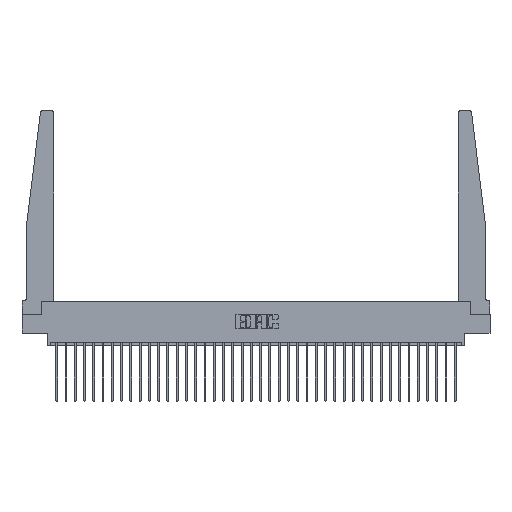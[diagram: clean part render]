
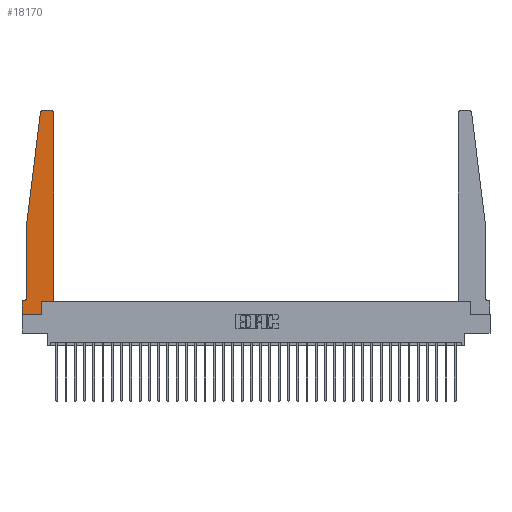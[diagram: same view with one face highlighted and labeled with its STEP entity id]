
A CAD part, top view. The second image highlights one B-rep face of the part: STEP entity #18170.
In plain terms, the highlighted planar face has unit normal (0, 0, 1).
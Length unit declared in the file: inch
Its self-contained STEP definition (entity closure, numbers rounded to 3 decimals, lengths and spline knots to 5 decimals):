
#316 = EDGE_CURVE ( 'NONE', #16473, #30556, #5155, .T. ) ;
#1388 = AXIS2_PLACEMENT_3D ( 'NONE', #4182, #32562, #17225 ) ;
#1612 = VECTOR ( 'NONE', #4434, 39.37008 ) ;
#2381 = ORIENTED_EDGE ( 'NONE', *, *, #28974, .T. ) ;
#2939 = CIRCLE ( 'NONE', #5296, 0.03 ) ;
#3600 = VERTEX_POINT ( 'NONE', #17891 ) ;
#3650 = CARTESIAN_POINT ( 'NONE',  ( 0., 0., 0.37 ) ) ;
#4142 = CARTESIAN_POINT ( 'NONE',  ( 0.425, 0.18, 0.37 ) ) ;
#4182 = CARTESIAN_POINT ( 'NONE',  ( 0., 0.1875, 0.37 ) ) ;
#4259 = VERTEX_POINT ( 'NONE', #17945 ) ;
#4434 = DIRECTION ( 'NONE',  ( -0.122, -0.992, 0. ) ) ;
#4478 = VECTOR ( 'NONE', #26945, 39.37008 ) ;
#4861 = EDGE_CURVE ( 'NONE', #17096, #24514, #8776, .T. ) ;
#5155 = LINE ( 'NONE', #4142, #24175 ) ;
#5296 = AXIS2_PLACEMENT_3D ( 'NONE', #6453, #24554, #9082 ) ;
#5481 = EDGE_CURVE ( 'NONE', #3600, #4259, #24488, .T. ) ;
#5769 = EDGE_CURVE ( 'NONE', #4259, #25946, #16413, .T. ) ;
#6453 = CARTESIAN_POINT ( 'NONE',  ( 0.27653, 2.72, 0.37 ) ) ;
#6488 = CARTESIAN_POINT ( 'NONE',  ( 0.015, 0.2375, 0.37 ) ) ;
#7365 = CARTESIAN_POINT ( 'NONE',  ( 0.425, 0.18, 0.37 ) ) ;
#7580 = DIRECTION ( 'NONE',  ( 0., -1., 0. ) ) ;
#7603 = EDGE_CURVE ( 'NONE', #23775, #3600, #21496, .T. ) ;
#7730 = VECTOR ( 'NONE', #19049, 39.37008 ) ;
#7959 = VECTOR ( 'NONE', #17327, 39.37008 ) ;
#8776 = LINE ( 'NONE', #9630, #7959 ) ;
#8950 = FACE_OUTER_BOUND ( 'NONE', #10271, .T. ) ;
#9082 = DIRECTION ( 'NONE',  ( 1., 0., 0. ) ) ;
#9118 = DIRECTION ( 'NONE',  ( -1., 0., 0. ) ) ;
#9524 = ORIENTED_EDGE ( 'NONE', *, *, #13020, .T. ) ;
#9630 = CARTESIAN_POINT ( 'NONE',  ( 0.25, 2.75, 0.37 ) ) ;
#9729 = VERTEX_POINT ( 'NONE', #31033 ) ;
#9930 = CARTESIAN_POINT ( 'NONE',  ( 0.395, 2.75, 0.37 ) ) ;
#10048 = ORIENTED_EDGE ( 'NONE', *, *, #7603, .T. ) ;
#10185 = DIRECTION ( 'NONE',  ( 0., 0., 1. ) ) ;
#10271 = EDGE_LOOP ( 'NONE', ( #30060, #20107, #10048, #21840, #12127, #16720, #18347, #21152, #9524, #21750, #13436, #2381 ) ) ;
#11219 = CARTESIAN_POINT ( 'NONE',  ( 0.425, 0.18, 0.37 ) ) ;
#11468 = LINE ( 'NONE', #7365, #24371 ) ;
#11501 = VECTOR ( 'NONE', #12660, 39.37008 ) ;
#11592 = VECTOR ( 'NONE', #14814, 39.37008 ) ;
#12127 = ORIENTED_EDGE ( 'NONE', *, *, #5769, .T. ) ;
#12216 = VERTEX_POINT ( 'NONE', #22411 ) ;
#12284 = CARTESIAN_POINT ( 'NONE',  ( 0.065, 1.25, 0.37 ) ) ;
#12615 = DIRECTION ( 'NONE',  ( 0., 1., 0. ) ) ;
#12660 = DIRECTION ( 'NONE',  ( 0., 1., 0. ) ) ;
#13020 = EDGE_CURVE ( 'NONE', #9729, #16473, #31198, .T. ) ;
#13436 = ORIENTED_EDGE ( 'NONE', *, *, #13509, .T. ) ;
#13509 = EDGE_CURVE ( 'NONE', #30556, #28440, #11468, .T. ) ;
#14289 = AXIS2_PLACEMENT_3D ( 'NONE', #6488, #24600, #9118 ) ;
#14741 = VECTOR ( 'NONE', #7580, 39.37008 ) ;
#14814 = DIRECTION ( 'NONE',  ( 0., -1., 0. ) ) ;
#16175 = CIRCLE ( 'NONE', #22724, 0.03 ) ;
#16204 = EDGE_CURVE ( 'NONE', #24514, #23775, #2939, .T. ) ;
#16413 = CIRCLE ( 'NONE', #14289, 0.05 ) ;
#16458 = CARTESIAN_POINT ( 'NONE',  ( 0.065, 0.1875, 0.37 ) ) ;
#16473 = VERTEX_POINT ( 'NONE', #33114 ) ;
#16503 = EDGE_CURVE ( 'NONE', #12216, #19919, #21583, .T. ) ;
#16720 = ORIENTED_EDGE ( 'NONE', *, *, #17979, .T. ) ;
#17096 = VERTEX_POINT ( 'NONE', #9930 ) ;
#17159 = CARTESIAN_POINT ( 'NONE',  ( 0.24675, 2.72367, 0.37 ) ) ;
#17225 = DIRECTION ( 'NONE',  ( 1., 0., 0. ) ) ;
#17327 = DIRECTION ( 'NONE',  ( -1., 0., 0. ) ) ;
#17891 = CARTESIAN_POINT ( 'NONE',  ( 0.065, 1.25, 0.37 ) ) ;
#17945 = CARTESIAN_POINT ( 'NONE',  ( 0.065, 0.2375, 0.37 ) ) ;
#17979 = EDGE_CURVE ( 'NONE', #25946, #12216, #28321, .T. ) ;
#18170 = ADVANCED_FACE ( 'NONE', ( #8950 ), #30014, .T. ) ;
#18347 = ORIENTED_EDGE ( 'NONE', *, *, #16503, .T. ) ;
#19049 = DIRECTION ( 'NONE',  ( -1., 0., 0. ) ) ;
#19919 = VERTEX_POINT ( 'NONE', #27713 ) ;
#20107 = ORIENTED_EDGE ( 'NONE', *, *, #16204, .T. ) ;
#20966 = CARTESIAN_POINT ( 'NONE',  ( 0.425, 2.72, 0.37 ) ) ;
#21152 = ORIENTED_EDGE ( 'NONE', *, *, #23638, .T. ) ;
#21496 = LINE ( 'NONE', #12284, #1612 ) ;
#21583 = LINE ( 'NONE', #30689, #14741 ) ;
#21750 = ORIENTED_EDGE ( 'NONE', *, *, #316, .T. ) ;
#21840 = ORIENTED_EDGE ( 'NONE', *, *, #5481, .T. ) ;
#22411 = CARTESIAN_POINT ( 'NONE',  ( 0., 0.1875, 0.37 ) ) ;
#22724 = AXIS2_PLACEMENT_3D ( 'NONE', #25641, #10185, #28212 ) ;
#23638 = EDGE_CURVE ( 'NONE', #19919, #9729, #25918, .T. ) ;
#23775 = VERTEX_POINT ( 'NONE', #17159 ) ;
#24175 = VECTOR ( 'NONE', #27422, 39.37008 ) ;
#24371 = VECTOR ( 'NONE', #12615, 39.37008 ) ;
#24488 = LINE ( 'NONE', #32726, #11592 ) ;
#24514 = VERTEX_POINT ( 'NONE', #28029 ) ;
#24554 = DIRECTION ( 'NONE',  ( 0., 0., 1. ) ) ;
#24600 = DIRECTION ( 'NONE',  ( 0., 0., -1. ) ) ;
#25641 = CARTESIAN_POINT ( 'NONE',  ( 0.395, 2.72, 0.37 ) ) ;
#25918 = LINE ( 'NONE', #3650, #4478 ) ;
#25946 = VERTEX_POINT ( 'NONE', #27584 ) ;
#26945 = DIRECTION ( 'NONE',  ( 1., 0., 0. ) ) ;
#27422 = DIRECTION ( 'NONE',  ( 1., 0., 0. ) ) ;
#27584 = CARTESIAN_POINT ( 'NONE',  ( 0.015, 0.1875, 0.37 ) ) ;
#27713 = CARTESIAN_POINT ( 'NONE',  ( 0., 0., 0.37 ) ) ;
#28029 = CARTESIAN_POINT ( 'NONE',  ( 0.27653, 2.75, 0.37 ) ) ;
#28074 = CARTESIAN_POINT ( 'NONE',  ( 0.2605, 0.18, 0.37 ) ) ;
#28212 = DIRECTION ( 'NONE',  ( 1., 0., 0. ) ) ;
#28321 = LINE ( 'NONE', #16458, #7730 ) ;
#28440 = VERTEX_POINT ( 'NONE', #20966 ) ;
#28974 = EDGE_CURVE ( 'NONE', #28440, #17096, #16175, .T. ) ;
#30014 = PLANE ( 'NONE',  #1388 ) ;
#30060 = ORIENTED_EDGE ( 'NONE', *, *, #4861, .T. ) ;
#30556 = VERTEX_POINT ( 'NONE', #11219 ) ;
#30689 = CARTESIAN_POINT ( 'NONE',  ( 0., 0., 0.37 ) ) ;
#31033 = CARTESIAN_POINT ( 'NONE',  ( 0.2605, 0., 0.37 ) ) ;
#31198 = LINE ( 'NONE', #28074, #11501 ) ;
#32562 = DIRECTION ( 'NONE',  ( 0., 0., 1. ) ) ;
#32726 = CARTESIAN_POINT ( 'NONE',  ( 0.065, 1.25, 0.37 ) ) ;
#33114 = CARTESIAN_POINT ( 'NONE',  ( 0.2605, 0.18, 0.37 ) ) ;
